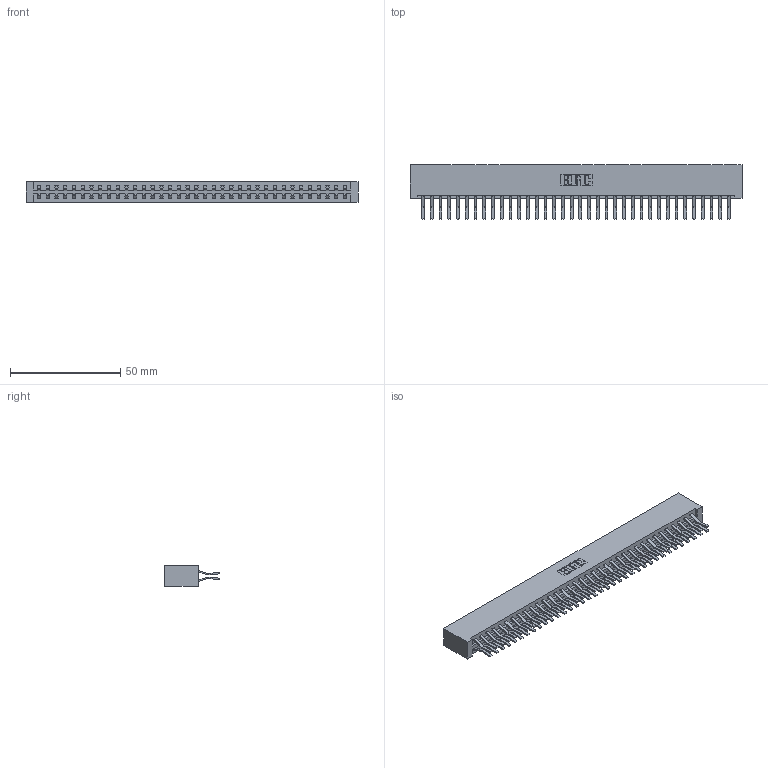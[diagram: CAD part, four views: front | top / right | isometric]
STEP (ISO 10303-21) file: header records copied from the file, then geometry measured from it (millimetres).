
FILE_DESCRIPTION (( 'STEP AP203' ), '1' );
FILE_NAME ('337-072-560-201.STEP', '2019-10-10T03:09:55', ( '' ), ( '' ), 'SwSTEP 2.0', 'SolidWorks 2016', '' );
FILE_SCHEMA (( 'CONFIG_CONTROL_DESIGN' ));
Length unit declared in the file: inch
Products named in the file (3): 345-292-001_560 Tail; 337-072-560-201; 337 Part_No Mounting Lugs
Assembly tree (73 placements, depth 2):
  337-072-560-201
    337 Part_No Mounting Lugs
    345-292-001_560 Tail  x72
Bounding box: 150.52 x 24.78 x 9.4 mm (x, y, z)
Volume: 17015.8 mm3; surface area: 20600.1 mm2
Topology: 73 solids, 73 shells, 4138 faces, 12311 edges, 8110 vertices
Faces by surface type: plane 2802, cylinder 1336
Entity records: 28499 total; most frequent: CARTESIAN_POINT 4806, ORIENTED_EDGE 4742, DIRECTION 4095, EDGE_CURVE 2371, VECTOR 2247, LINE 2247, VERTEX_POINT 1578, AXIS2_PLACEMENT_3D 924
